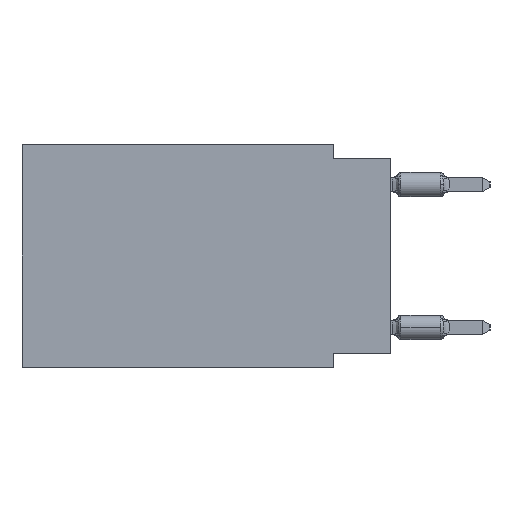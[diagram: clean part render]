
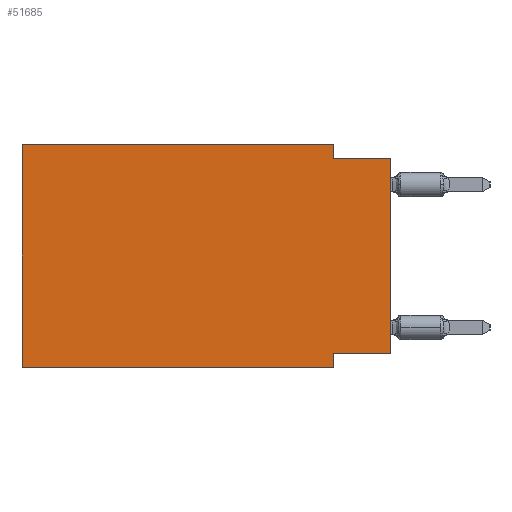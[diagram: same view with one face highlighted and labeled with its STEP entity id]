
A CAD part, left-side view. The second image highlights one B-rep face of the part: STEP entity #51685.
In plain terms, the highlighted planar face has unit normal (-1, 0, 0).
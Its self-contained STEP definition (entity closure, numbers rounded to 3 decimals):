
#287 = ORIENTED_EDGE ( 'NONE', *, *, #40946, .F. ) ;
#462 = LINE ( 'NONE', #41181, #27064 ) ;
#665 = VECTOR ( 'NONE', #41594, 1000. ) ;
#1515 = LINE ( 'NONE', #28553, #62392 ) ;
#2624 = PLANE ( 'NONE',  #35472 ) ;
#3036 = DIRECTION ( 'NONE',  ( 0., -1., 0. ) ) ;
#4771 = LINE ( 'NONE', #52292, #47203 ) ;
#5213 = VERTEX_POINT ( 'NONE', #65839 ) ;
#5437 = DIRECTION ( 'NONE',  ( 0., 0., 1. ) ) ;
#5726 = ORIENTED_EDGE ( 'NONE', *, *, #51491, .F. ) ;
#6491 = CARTESIAN_POINT ( 'NONE',  ( 0., 2.54, -9.271 ) ) ;
#7454 = EDGE_CURVE ( 'NONE', #38250, #15772, #4771, .T. ) ;
#11696 = LINE ( 'NONE', #65609, #27670 ) ;
#11962 = VERTEX_POINT ( 'NONE', #6491 ) ;
#12627 = EDGE_CURVE ( 'NONE', #5213, #15786, #21525, .T. ) ;
#13872 = EDGE_CURVE ( 'NONE', #15772, #18781, #11696, .T. ) ;
#14175 = LINE ( 'NONE', #49778, #31427 ) ;
#14647 = CARTESIAN_POINT ( 'NONE',  ( 0., 2.54, -0.635 ) ) ;
#15772 = VERTEX_POINT ( 'NONE', #14647 ) ;
#15786 = VERTEX_POINT ( 'NONE', #63765 ) ;
#16990 = VECTOR ( 'NONE', #18586, 1000. ) ;
#18034 = DIRECTION ( 'NONE',  ( 0., 0., -1. ) ) ;
#18586 = DIRECTION ( 'NONE',  ( 0., -1., 0. ) ) ;
#18781 = VERTEX_POINT ( 'NONE', #21335 ) ;
#19337 = DIRECTION ( 'NONE',  ( 0., 1., 0. ) ) ;
#20427 = LINE ( 'NONE', #41276, #665 ) ;
#21335 = CARTESIAN_POINT ( 'NONE',  ( 0., 0., -0.635 ) ) ;
#21343 = DIRECTION ( 'NONE',  ( 0., -1., 0. ) ) ;
#21525 = LINE ( 'NONE', #52278, #61707 ) ;
#22209 = ORIENTED_EDGE ( 'NONE', *, *, #13872, .F. ) ;
#22945 = ORIENTED_EDGE ( 'NONE', *, *, #7454, .F. ) ;
#23781 = CARTESIAN_POINT ( 'NONE',  ( 0., 2.54, 0. ) ) ;
#23970 = VERTEX_POINT ( 'NONE', #40905 ) ;
#25733 = EDGE_CURVE ( 'NONE', #15786, #38250, #44569, .T. ) ;
#27064 = VECTOR ( 'NONE', #21343, 1000. ) ;
#27670 = VECTOR ( 'NONE', #3036, 1000. ) ;
#28553 = CARTESIAN_POINT ( 'NONE',  ( 0., 0., 0. ) ) ;
#29312 = CARTESIAN_POINT ( 'NONE',  ( 0., 16.383, 0. ) ) ;
#29345 = ORIENTED_EDGE ( 'NONE', *, *, #47412, .T. ) ;
#31427 = VECTOR ( 'NONE', #19337, 1000. ) ;
#34441 = DIRECTION ( 'NONE',  ( 1., 0., 0. ) ) ;
#35472 = AXIS2_PLACEMENT_3D ( 'NONE', #29312, #34441, #18034 ) ;
#38250 = VERTEX_POINT ( 'NONE', #23781 ) ;
#40905 = CARTESIAN_POINT ( 'NONE',  ( 0., 2.54, -9.906 ) ) ;
#40946 = EDGE_CURVE ( 'NONE', #64485, #11962, #14175, .T. ) ;
#41099 = EDGE_CURVE ( 'NONE', #5213, #23970, #462, .T. ) ;
#41181 = CARTESIAN_POINT ( 'NONE',  ( 0., 16.383, -9.906 ) ) ;
#41276 = CARTESIAN_POINT ( 'NONE',  ( 0., 2.54, -9.906 ) ) ;
#41594 = DIRECTION ( 'NONE',  ( 0., 0., -1. ) ) ;
#42286 = ORIENTED_EDGE ( 'NONE', *, *, #12627, .F. ) ;
#43214 = CARTESIAN_POINT ( 'NONE',  ( 0., 16.383, 0. ) ) ;
#43576 = DIRECTION ( 'NONE',  ( 0., 0., 1. ) ) ;
#43843 = CARTESIAN_POINT ( 'NONE',  ( 0., 0., -9.271 ) ) ;
#44569 = LINE ( 'NONE', #43214, #16990 ) ;
#46501 = DIRECTION ( 'NONE',  ( 0., 0., -1. ) ) ;
#47203 = VECTOR ( 'NONE', #46501, 1000. ) ;
#47412 = EDGE_CURVE ( 'NONE', #64485, #18781, #1515, .T. ) ;
#49778 = CARTESIAN_POINT ( 'NONE',  ( 0., 0., -9.271 ) ) ;
#51491 = EDGE_CURVE ( 'NONE', #11962, #23970, #20427, .T. ) ;
#51685 = ADVANCED_FACE ( 'NONE', ( #60404 ), #2624, .F. ) ;
#52278 = CARTESIAN_POINT ( 'NONE',  ( 0., 16.383, 0. ) ) ;
#52292 = CARTESIAN_POINT ( 'NONE',  ( 0., 2.54, 0. ) ) ;
#58853 = EDGE_LOOP ( 'NONE', ( #29345, #22209, #22945, #62323, #42286, #59027, #5726, #287 ) ) ;
#59027 = ORIENTED_EDGE ( 'NONE', *, *, #41099, .T. ) ;
#60404 = FACE_OUTER_BOUND ( 'NONE', #58853, .T. ) ;
#61707 = VECTOR ( 'NONE', #5437, 1000. ) ;
#62323 = ORIENTED_EDGE ( 'NONE', *, *, #25733, .F. ) ;
#62392 = VECTOR ( 'NONE', #43576, 1000. ) ;
#63765 = CARTESIAN_POINT ( 'NONE',  ( 0., 16.383, 0. ) ) ;
#64485 = VERTEX_POINT ( 'NONE', #43843 ) ;
#65609 = CARTESIAN_POINT ( 'NONE',  ( 0., 0., -0.635 ) ) ;
#65839 = CARTESIAN_POINT ( 'NONE',  ( 0., 16.383, -9.906 ) ) ;
